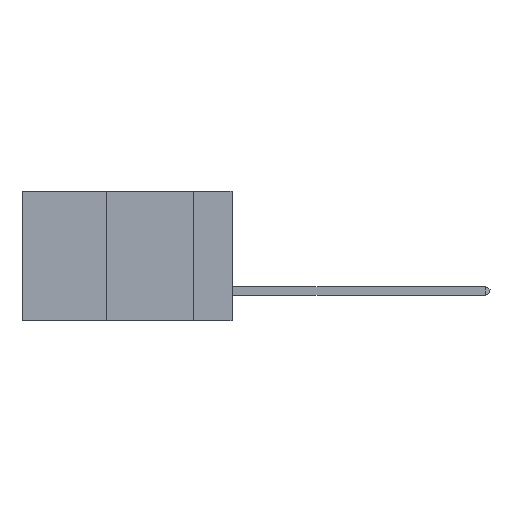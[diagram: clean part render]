
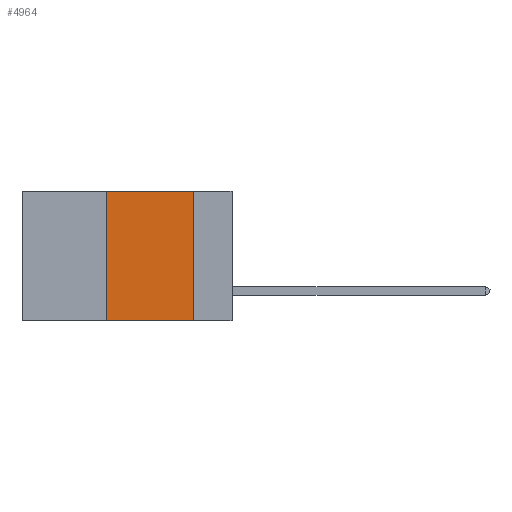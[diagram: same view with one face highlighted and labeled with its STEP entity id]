
A CAD part, left-side view. The second image highlights one B-rep face of the part: STEP entity #4964.
In plain terms, the highlighted planar face has unit normal (-1, 0, 0).
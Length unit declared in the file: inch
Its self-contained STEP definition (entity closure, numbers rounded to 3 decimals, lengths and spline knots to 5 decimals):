
#300 = DIRECTION ( 'NONE',  ( 0., 0., -1. ) ) ;
#435 = LINE ( 'NONE', #3588, #12448 ) ;
#590 = VERTEX_POINT ( 'NONE', #12671 ) ;
#742 = EDGE_CURVE ( 'NONE', #6454, #8194, #435, .T. ) ;
#780 = EDGE_LOOP ( 'NONE', ( #12832, #12100, #9719, #8281 ) ) ;
#1413 = DIRECTION ( 'NONE',  ( 0., -1., 0. ) ) ;
#1710 = LINE ( 'NONE', #2320, #11226 ) ;
#2320 = CARTESIAN_POINT ( 'NONE',  ( 0., 0.6, 0. ) ) ;
#3007 = EDGE_CURVE ( 'NONE', #590, #5308, #12538, .T. ) ;
#3588 = CARTESIAN_POINT ( 'NONE',  ( 0., 0.11, 0. ) ) ;
#4620 = DIRECTION ( 'NONE',  ( 1., 0., 0. ) ) ;
#4964 = ADVANCED_FACE ( 'NONE', ( #8984 ), #11151, .F. ) ;
#5187 = AXIS2_PLACEMENT_3D ( 'NONE', #6670, #4620, #300 ) ;
#5308 = VERTEX_POINT ( 'NONE', #10764 ) ;
#5721 = CARTESIAN_POINT ( 'NONE',  ( 0., 0.6, -0.37 ) ) ;
#6177 = VECTOR ( 'NONE', #9657, 39.37008 ) ;
#6454 = VERTEX_POINT ( 'NONE', #6668 ) ;
#6535 = CARTESIAN_POINT ( 'NONE',  ( 0., 0.36, 0. ) ) ;
#6668 = CARTESIAN_POINT ( 'NONE',  ( 0., 0.11, 0. ) ) ;
#6670 = CARTESIAN_POINT ( 'NONE',  ( 0., 0.6, 0. ) ) ;
#6904 = EDGE_CURVE ( 'NONE', #5308, #6454, #1710, .T. ) ;
#7051 = EDGE_CURVE ( 'NONE', #590, #8194, #8709, .T. ) ;
#8072 = CARTESIAN_POINT ( 'NONE',  ( 0., 0.11, -0.37 ) ) ;
#8194 = VERTEX_POINT ( 'NONE', #8072 ) ;
#8281 = ORIENTED_EDGE ( 'NONE', *, *, #7051, .T. ) ;
#8709 = LINE ( 'NONE', #5721, #10881 ) ;
#8710 = DIRECTION ( 'NONE',  ( 0., 0., -1. ) ) ;
#8984 = FACE_OUTER_BOUND ( 'NONE', #780, .T. ) ;
#9657 = DIRECTION ( 'NONE',  ( 0., 0., 1. ) ) ;
#9719 = ORIENTED_EDGE ( 'NONE', *, *, #3007, .F. ) ;
#9796 = DIRECTION ( 'NONE',  ( 0., -1., 0. ) ) ;
#10764 = CARTESIAN_POINT ( 'NONE',  ( 0., 0.36, 0. ) ) ;
#10881 = VECTOR ( 'NONE', #1413, 39.37008 ) ;
#11151 = PLANE ( 'NONE',  #5187 ) ;
#11226 = VECTOR ( 'NONE', #9796, 39.37008 ) ;
#12100 = ORIENTED_EDGE ( 'NONE', *, *, #6904, .F. ) ;
#12448 = VECTOR ( 'NONE', #8710, 39.37008 ) ;
#12538 = LINE ( 'NONE', #6535, #6177 ) ;
#12671 = CARTESIAN_POINT ( 'NONE',  ( 0., 0.36, -0.37 ) ) ;
#12832 = ORIENTED_EDGE ( 'NONE', *, *, #742, .F. ) ;
